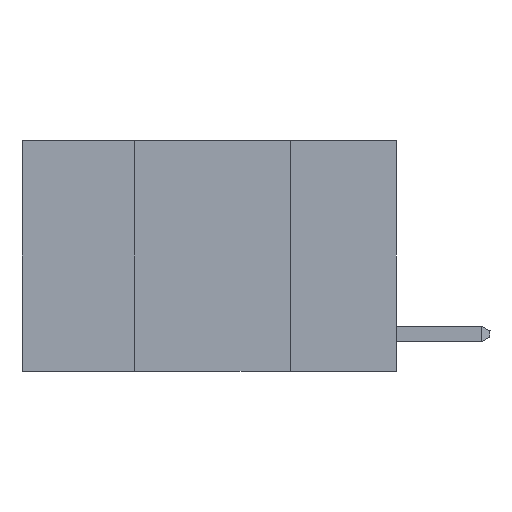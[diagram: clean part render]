
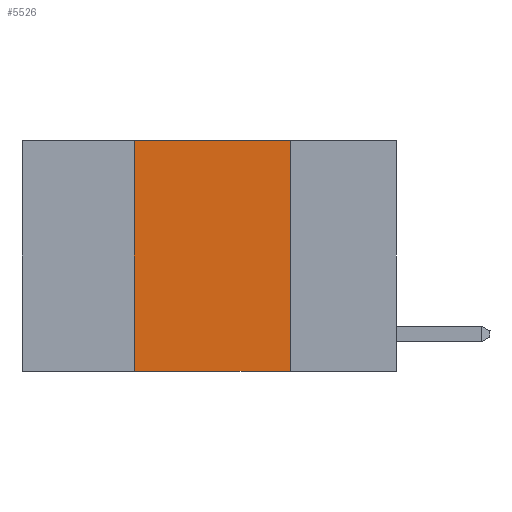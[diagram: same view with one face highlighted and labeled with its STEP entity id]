
A CAD part, left-side view. The second image highlights one B-rep face of the part: STEP entity #5526.
In plain terms, the highlighted planar face has unit normal (-1, 0, 0).
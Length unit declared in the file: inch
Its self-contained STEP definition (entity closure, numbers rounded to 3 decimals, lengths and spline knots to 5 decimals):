
#485 = ORIENTED_EDGE ( 'NONE', *, *, #5061, .F. ) ;
#1144 = VERTEX_POINT ( 'NONE', #1426 ) ;
#1286 = CARTESIAN_POINT ( 'NONE',  ( 0., 0.42, -0.37 ) ) ;
#1426 = CARTESIAN_POINT ( 'NONE',  ( 0., 0.17, -0.37 ) ) ;
#1450 = DIRECTION ( 'NONE',  ( 1., 0., 0. ) ) ;
#1531 = DIRECTION ( 'NONE',  ( 0., 0., -1. ) ) ;
#1602 = CARTESIAN_POINT ( 'NONE',  ( 0., 0.6, 0. ) ) ;
#1690 = EDGE_CURVE ( 'NONE', #2900, #7865, #8778, .T. ) ;
#2593 = ORIENTED_EDGE ( 'NONE', *, *, #5777, .F. ) ;
#2900 = VERTEX_POINT ( 'NONE', #1286 ) ;
#3141 = EDGE_LOOP ( 'NONE', ( #2593, #485, #11137, #6747 ) ) ;
#3634 = VERTEX_POINT ( 'NONE', #9240 ) ;
#3846 = VECTOR ( 'NONE', #4485, 39.37008 ) ;
#4081 = AXIS2_PLACEMENT_3D ( 'NONE', #1602, #1450, #1531 ) ;
#4305 = PLANE ( 'NONE',  #4081 ) ;
#4485 = DIRECTION ( 'NONE',  ( 0., -1., 0. ) ) ;
#4576 = CARTESIAN_POINT ( 'NONE',  ( 0., 0.6, -0.37 ) ) ;
#5061 = EDGE_CURVE ( 'NONE', #7865, #3634, #11801, .T. ) ;
#5103 = DIRECTION ( 'NONE',  ( 0., -1., 0. ) ) ;
#5526 = ADVANCED_FACE ( 'NONE', ( #7906 ), #4305, .F. ) ;
#5777 = EDGE_CURVE ( 'NONE', #3634, #1144, #6647, .T. ) ;
#5806 = VECTOR ( 'NONE', #6202, 39.37008 ) ;
#6202 = DIRECTION ( 'NONE',  ( 0., 0., -1. ) ) ;
#6531 = VECTOR ( 'NONE', #5103, 39.37008 ) ;
#6622 = DIRECTION ( 'NONE',  ( 0., 0., 1. ) ) ;
#6647 = LINE ( 'NONE', #10821, #5806 ) ;
#6747 = ORIENTED_EDGE ( 'NONE', *, *, #9306, .T. ) ;
#7819 = CARTESIAN_POINT ( 'NONE',  ( 0., 0.6, 0. ) ) ;
#7865 = VERTEX_POINT ( 'NONE', #8787 ) ;
#7906 = FACE_OUTER_BOUND ( 'NONE', #3141, .T. ) ;
#7912 = CARTESIAN_POINT ( 'NONE',  ( 0., 0.42, 0. ) ) ;
#8049 = VECTOR ( 'NONE', #6622, 39.37008 ) ;
#8778 = LINE ( 'NONE', #7912, #8049 ) ;
#8787 = CARTESIAN_POINT ( 'NONE',  ( 0., 0.42, 0. ) ) ;
#9240 = CARTESIAN_POINT ( 'NONE',  ( 0., 0.17, 0. ) ) ;
#9306 = EDGE_CURVE ( 'NONE', #2900, #1144, #11417, .T. ) ;
#10821 = CARTESIAN_POINT ( 'NONE',  ( 0., 0.17, 0. ) ) ;
#11137 = ORIENTED_EDGE ( 'NONE', *, *, #1690, .F. ) ;
#11417 = LINE ( 'NONE', #4576, #3846 ) ;
#11801 = LINE ( 'NONE', #7819, #6531 ) ;
